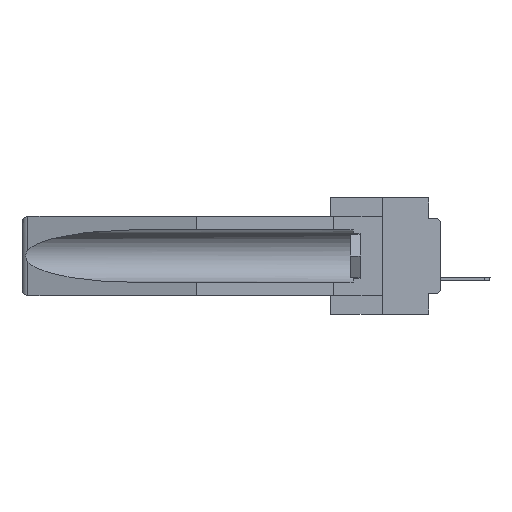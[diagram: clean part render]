
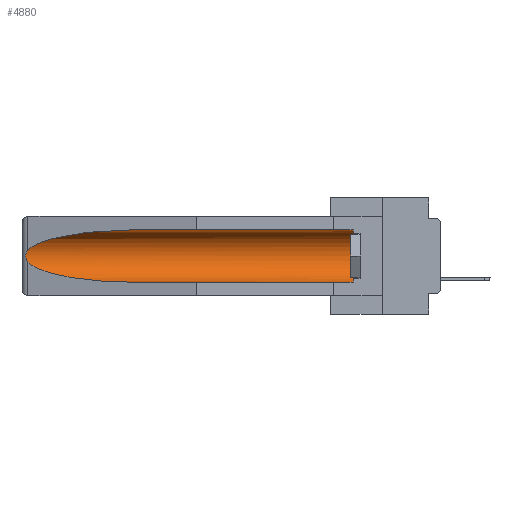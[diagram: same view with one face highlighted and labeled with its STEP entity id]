
A CAD part, left-side view. The second image highlights one B-rep face of the part: STEP entity #4880.
In plain terms, the highlighted cylindrical face has radius 2.857 mm (diameter 5.715 mm), a partial arc.
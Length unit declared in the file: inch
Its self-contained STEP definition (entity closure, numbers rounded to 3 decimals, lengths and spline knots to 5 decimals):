
#349 = CARTESIAN_POINT ( 'NONE',  ( 0.155, 1.07973, -0.059 ) ) ;
#446 = CARTESIAN_POINT ( 'NONE',  ( 0.25451, 1.48313, -0.09465 ) ) ;
#619 = CARTESIAN_POINT ( 'NONE',  ( 0.155, 1.07973, -0.284 ) ) ;
#1721 = AXIS2_PLACEMENT_3D ( 'NONE', #36668, #15672, #18916 ) ;
#1789 = CARTESIAN_POINT ( 'NONE',  ( 0.26655, 1.53094, -0.18657 ) ) ;
#3523 = CARTESIAN_POINT ( 'NONE',  ( 0.25451, 1.48313, -0.24835 ) ) ;
#3808 = VECTOR ( 'NONE', #9355, 39.37008 ) ;
#4046 = CARTESIAN_POINT ( 'NONE',  ( 0.21114, 1.30732, -0.284 ) ) ;
#4726 = CARTESIAN_POINT ( 'NONE',  ( 0.155, -0.30754, -0.1715 ) ) ;
#4880 = ADVANCED_FACE ( 'NONE', ( #23530 ), #14228, .F. ) ;
#5521 = VERTEX_POINT ( 'NONE', #25664 ) ;
#5793 =( BOUNDED_CURVE ( )  B_SPLINE_CURVE ( 3, ( #27765, #3523, #4046, #619 ),
 .UNSPECIFIED., .F., .F. ) 
 B_SPLINE_CURVE_WITH_KNOTS ( ( 4, 4 ),
 ( 0.1948, 1.5708 ),
 .UNSPECIFIED. ) 
 CURVE ( )  GEOMETRIC_REPRESENTATION_ITEM ( )  RATIONAL_B_SPLINE_CURVE ( ( 1., 0.848, 0.848, 1. ) ) 
 REPRESENTATION_ITEM ( '' )  );
#5942 = EDGE_CURVE ( 'NONE', #28925, #15782, #13112, .T. ) ;
#7252 = CARTESIAN_POINT ( 'NONE',  ( 0.2673, 1.53269, -0.17917 ) ) ;
#8519 = CARTESIAN_POINT ( 'NONE',  ( 0.155, 0.126, -0.059 ) ) ;
#9355 = DIRECTION ( 'NONE',  ( 0., 1., 0. ) ) ;
#10095 = EDGE_CURVE ( 'NONE', #13166, #28925, #36022, .T. ) ;
#10098 = DIRECTION ( 'NONE',  ( 0., 0., 1. ) ) ;
#10325 = CARTESIAN_POINT ( 'NONE',  ( 0.2673, 1.5327, -0.16383 ) ) ;
#13112 = LINE ( 'NONE', #30381, #3808 ) ;
#13166 = VERTEX_POINT ( 'NONE', #36828 ) ;
#13604 = CARTESIAN_POINT ( 'NONE',  ( 0.26597, 1.52961, -0.15275 ) ) ;
#14228 = CYLINDRICAL_SURFACE ( 'NONE', #26505, 0.1125 ) ;
#14234 = CARTESIAN_POINT ( 'NONE',  ( 0.26537, 1.52718, -0.19328 ) ) ;
#15672 = DIRECTION ( 'NONE',  ( 0., -1., 0. ) ) ;
#15767 = ORIENTED_EDGE ( 'NONE', *, *, #29374, .T. ) ;
#15782 = VERTEX_POINT ( 'NONE', #24985 ) ;
#16610 = CARTESIAN_POINT ( 'NONE',  ( 0.26597, 1.5296, -0.19026 ) ) ;
#17169 = EDGE_CURVE ( 'NONE', #25220, #28297, #5793, .T. ) ;
#17920 = CARTESIAN_POINT ( 'NONE',  ( 0.26537, 1.52718, -0.14972 ) ) ;
#18269 = ORIENTED_EDGE ( 'NONE', *, *, #10095, .T. ) ;
#18916 = DIRECTION ( 'NONE',  ( 0., 0., 1. ) ) ;
#21742 = ORIENTED_EDGE ( 'NONE', *, *, #37868, .T. ) ;
#22175 = CARTESIAN_POINT ( 'NONE',  ( 0.2675, 1.53308, -0.16763 ) ) ;
#23012 = ORIENTED_EDGE ( 'NONE', *, *, #26494, .F. ) ;
#23530 = FACE_OUTER_BOUND ( 'NONE', #29888, .T. ) ;
#23944 = CARTESIAN_POINT ( 'NONE',  ( 0.155, -0.30754, -0.284 ) ) ;
#24985 = CARTESIAN_POINT ( 'NONE',  ( 0.155, 1.07973, -0.059 ) ) ;
#25134 = ORIENTED_EDGE ( 'NONE', *, *, #5942, .T. ) ;
#25220 = VERTEX_POINT ( 'NONE', #14234 ) ;
#25416 = CARTESIAN_POINT ( 'NONE',  ( 0.26537, 1.52718, -0.14972 ) ) ;
#25664 = CARTESIAN_POINT ( 'NONE',  ( 0.26537, 1.52718, -0.14972 ) ) ;
#26027 = VECTOR ( 'NONE', #30003, 39.37008 ) ;
#26494 = EDGE_CURVE ( 'NONE', #13166, #28297, #32909, .T. ) ;
#26505 = AXIS2_PLACEMENT_3D ( 'NONE', #4726, #31416, #10098 ) ;
#27765 = CARTESIAN_POINT ( 'NONE',  ( 0.26537, 1.52718, -0.19328 ) ) ;
#28297 = VERTEX_POINT ( 'NONE', #32617 ) ;
#28925 = VERTEX_POINT ( 'NONE', #8519 ) ;
#29374 = EDGE_CURVE ( 'NONE', #15782, #5521, #31146, .T. ) ;
#29888 = EDGE_LOOP ( 'NONE', ( #15767, #21742, #33139, #23012, #18269, #25134 ) ) ;
#30003 = DIRECTION ( 'NONE',  ( 0., 1., 0. ) ) ;
#30381 = CARTESIAN_POINT ( 'NONE',  ( 0.155, -0.30754, -0.059 ) ) ;
#30420 = B_SPLINE_CURVE_WITH_KNOTS ( 'NONE', 3,
 ( #25416, #13604, #34362, #10325, #22175, #31515, #7252, #1789, #16610, #31106 ),
 .UNSPECIFIED., .F., .F.,
 ( 4, 2, 2, 2, 4 ),
 ( 0., 0.00029, 0.00058, 0.00087, 0.00117 ),
 .UNSPECIFIED. ) ;
#31106 = CARTESIAN_POINT ( 'NONE',  ( 0.26537, 1.52718, -0.19328 ) ) ;
#31146 =( BOUNDED_CURVE ( )  B_SPLINE_CURVE ( 3, ( #349, #33159, #446, #17920 ),
 .UNSPECIFIED., .F., .F. ) 
 B_SPLINE_CURVE_WITH_KNOTS ( ( 4, 4 ),
 ( 4.71239, 6.08839 ),
 .UNSPECIFIED. ) 
 CURVE ( )  GEOMETRIC_REPRESENTATION_ITEM ( )  RATIONAL_B_SPLINE_CURVE ( ( 1., 0.848, 0.848, 1. ) ) 
 REPRESENTATION_ITEM ( '' )  );
#31416 = DIRECTION ( 'NONE',  ( 0., 1., 0. ) ) ;
#31515 = CARTESIAN_POINT ( 'NONE',  ( 0.2675, 1.53308, -0.17534 ) ) ;
#32617 = CARTESIAN_POINT ( 'NONE',  ( 0.155, 1.07973, -0.284 ) ) ;
#32909 = LINE ( 'NONE', #23944, #26027 ) ;
#33139 = ORIENTED_EDGE ( 'NONE', *, *, #17169, .T. ) ;
#33159 = CARTESIAN_POINT ( 'NONE',  ( 0.21114, 1.30732, -0.059 ) ) ;
#34362 = CARTESIAN_POINT ( 'NONE',  ( 0.26654, 1.53092, -0.15636 ) ) ;
#36022 = CIRCLE ( 'NONE', #1721, 0.1125 ) ;
#36668 = CARTESIAN_POINT ( 'NONE',  ( 0.155, 0.126, -0.1715 ) ) ;
#36828 = CARTESIAN_POINT ( 'NONE',  ( 0.155, 0.126, -0.284 ) ) ;
#37868 = EDGE_CURVE ( 'NONE', #5521, #25220, #30420, .T. ) ;
